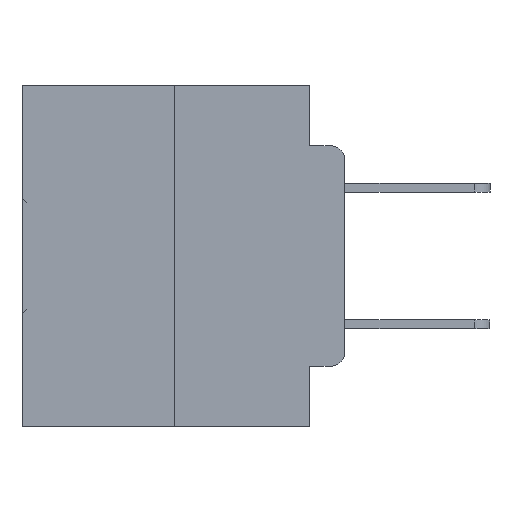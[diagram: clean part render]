
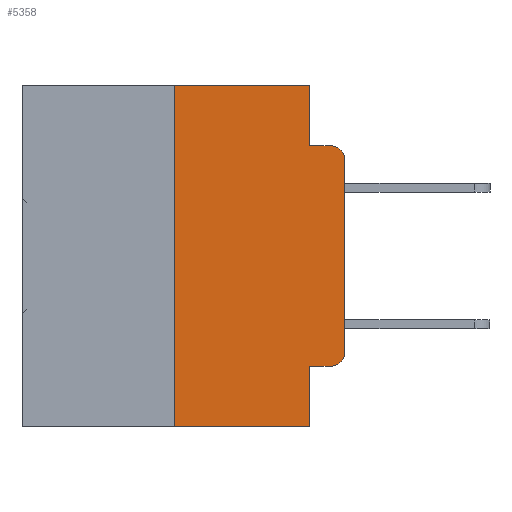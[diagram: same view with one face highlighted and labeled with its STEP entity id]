
A CAD part, left-side view. The second image highlights one B-rep face of the part: STEP entity #5358.
In plain terms, the highlighted planar face has unit normal (-1, 0, 0).
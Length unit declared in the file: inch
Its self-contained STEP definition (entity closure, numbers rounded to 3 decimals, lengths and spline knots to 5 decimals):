
#690 = CARTESIAN_POINT ( 'NONE',  ( 0., 0.051, -0.4115 ) ) ;
#1845 = DIRECTION ( 'NONE',  ( 0., -1., 0. ) ) ;
#2079 = CARTESIAN_POINT ( 'NONE',  ( 0., 0.25, -0.5 ) ) ;
#2485 = ORIENTED_EDGE ( 'NONE', *, *, #14139, .T. ) ;
#2536 = DIRECTION ( 'NONE',  ( 1., 0., 0. ) ) ;
#2561 = VERTEX_POINT ( 'NONE', #8249 ) ;
#4065 = LINE ( 'NONE', #8374, #10521 ) ;
#4293 = DIRECTION ( 'NONE',  ( 0., 0., 1. ) ) ;
#5358 = ADVANCED_FACE ( 'NONE', ( #15843 ), #18816, .F. ) ;
#5550 = AXIS2_PLACEMENT_3D ( 'NONE', #29505, #2536, #21541 ) ;
#5890 = CARTESIAN_POINT ( 'NONE',  ( 0., 0.051, -0.0885 ) ) ;
#6060 = EDGE_CURVE ( 'NONE', #31993, #30257, #15379, .T. ) ;
#6464 = VERTEX_POINT ( 'NONE', #7385 ) ;
#7130 = CIRCLE ( 'NONE', #8031, 0.02 ) ;
#7385 = CARTESIAN_POINT ( 'NONE',  ( 0., 0.051, -0.5 ) ) ;
#7533 = VECTOR ( 'NONE', #12114, 39.37008 ) ;
#8031 = AXIS2_PLACEMENT_3D ( 'NONE', #27682, #11628, #30417 ) ;
#8249 = CARTESIAN_POINT ( 'NONE',  ( 0., 0.02, -0.4115 ) ) ;
#8374 = CARTESIAN_POINT ( 'NONE',  ( 0., 0.473, 0. ) ) ;
#8397 = LINE ( 'NONE', #14814, #7533 ) ;
#8504 = ORIENTED_EDGE ( 'NONE', *, *, #6060, .F. ) ;
#9552 = EDGE_CURVE ( 'NONE', #32335, #24840, #14084, .T. ) ;
#10448 = EDGE_CURVE ( 'NONE', #24156, #6464, #14868, .T. ) ;
#10521 = VECTOR ( 'NONE', #29969, 39.37008 ) ;
#11304 = CARTESIAN_POINT ( 'NONE',  ( 0., 0.25, 0. ) ) ;
#11628 = DIRECTION ( 'NONE',  ( -1., 0., 0. ) ) ;
#11747 = CARTESIAN_POINT ( 'NONE',  ( 0., 0.02, -0.1085 ) ) ;
#11775 = AXIS2_PLACEMENT_3D ( 'NONE', #11747, #30529, #14446 ) ;
#11780 = VERTEX_POINT ( 'NONE', #16241 ) ;
#11903 = CARTESIAN_POINT ( 'NONE',  ( 0., 0.051, 0. ) ) ;
#12114 = DIRECTION ( 'NONE',  ( 0., 0., -1. ) ) ;
#12718 = CARTESIAN_POINT ( 'NONE',  ( 0., 0., 0. ) ) ;
#14007 = DIRECTION ( 'NONE',  ( 0., 0., 1. ) ) ;
#14016 = CARTESIAN_POINT ( 'NONE',  ( 0., 0., -0.1085 ) ) ;
#14084 = LINE ( 'NONE', #20851, #34625 ) ;
#14139 = EDGE_CURVE ( 'NONE', #20194, #27164, #27593, .T. ) ;
#14446 = DIRECTION ( 'NONE',  ( 0., 0., -1. ) ) ;
#14524 = ORIENTED_EDGE ( 'NONE', *, *, #17214, .T. ) ;
#14561 = VECTOR ( 'NONE', #33885, 39.37008 ) ;
#14765 = EDGE_CURVE ( 'NONE', #24156, #2561, #21674, .T. ) ;
#14814 = CARTESIAN_POINT ( 'NONE',  ( 0., 0.051, 0. ) ) ;
#14868 = LINE ( 'NONE', #11903, #29979 ) ;
#15379 = LINE ( 'NONE', #11304, #22541 ) ;
#15843 = FACE_OUTER_BOUND ( 'NONE', #30487, .T. ) ;
#16241 = CARTESIAN_POINT ( 'NONE',  ( 0., 0.051, 0. ) ) ;
#17214 = EDGE_CURVE ( 'NONE', #2561, #20194, #7130, .T. ) ;
#17261 = EDGE_CURVE ( 'NONE', #27164, #24840, #27839, .T. ) ;
#17443 = ORIENTED_EDGE ( 'NONE', *, *, #21713, .T. ) ;
#17823 = DIRECTION ( 'NONE',  ( 0., -1., 0. ) ) ;
#18374 = EDGE_CURVE ( 'NONE', #30257, #11780, #4065, .T. ) ;
#18658 = ORIENTED_EDGE ( 'NONE', *, *, #9552, .F. ) ;
#18816 = PLANE ( 'NONE',  #5550 ) ;
#20194 = VERTEX_POINT ( 'NONE', #26821 ) ;
#20476 = VECTOR ( 'NONE', #4293, 39.37008 ) ;
#20851 = CARTESIAN_POINT ( 'NONE',  ( 0., 0.051, -0.0885 ) ) ;
#21541 = DIRECTION ( 'NONE',  ( 0., 0., -1. ) ) ;
#21674 = LINE ( 'NONE', #31210, #14561 ) ;
#21713 = EDGE_CURVE ( 'NONE', #31993, #6464, #34153, .T. ) ;
#22064 = ORIENTED_EDGE ( 'NONE', *, *, #18374, .F. ) ;
#22541 = VECTOR ( 'NONE', #14007, 39.37008 ) ;
#22568 = DIRECTION ( 'NONE',  ( 0., 0., -1. ) ) ;
#24142 = ORIENTED_EDGE ( 'NONE', *, *, #17261, .T. ) ;
#24156 = VERTEX_POINT ( 'NONE', #690 ) ;
#24840 = VERTEX_POINT ( 'NONE', #33296 ) ;
#26632 = ORIENTED_EDGE ( 'NONE', *, *, #33195, .F. ) ;
#26821 = CARTESIAN_POINT ( 'NONE',  ( 0., 0., -0.3915 ) ) ;
#27164 = VERTEX_POINT ( 'NONE', #14016 ) ;
#27593 = LINE ( 'NONE', #12718, #20476 ) ;
#27682 = CARTESIAN_POINT ( 'NONE',  ( 0., 0.02, -0.3915 ) ) ;
#27839 = CIRCLE ( 'NONE', #11775, 0.02 ) ;
#27926 = ORIENTED_EDGE ( 'NONE', *, *, #14765, .T. ) ;
#29505 = CARTESIAN_POINT ( 'NONE',  ( 0., 0.473, 0. ) ) ;
#29969 = DIRECTION ( 'NONE',  ( 0., -1., 0. ) ) ;
#29979 = VECTOR ( 'NONE', #22568, 39.37008 ) ;
#30257 = VERTEX_POINT ( 'NONE', #30896 ) ;
#30417 = DIRECTION ( 'NONE',  ( 0., 0., -1. ) ) ;
#30487 = EDGE_LOOP ( 'NONE', ( #2485, #24142, #18658, #26632, #22064, #8504, #17443, #32542, #27926, #14524 ) ) ;
#30529 = DIRECTION ( 'NONE',  ( -1., 0., 0. ) ) ;
#30896 = CARTESIAN_POINT ( 'NONE',  ( 0., 0.25, 0. ) ) ;
#31210 = CARTESIAN_POINT ( 'NONE',  ( 0., 0.051, -0.4115 ) ) ;
#31236 = CARTESIAN_POINT ( 'NONE',  ( 0., 0.473, -0.5 ) ) ;
#31993 = VERTEX_POINT ( 'NONE', #2079 ) ;
#32335 = VERTEX_POINT ( 'NONE', #5890 ) ;
#32542 = ORIENTED_EDGE ( 'NONE', *, *, #10448, .F. ) ;
#33195 = EDGE_CURVE ( 'NONE', #11780, #32335, #8397, .T. ) ;
#33296 = CARTESIAN_POINT ( 'NONE',  ( 0., 0.02, -0.0885 ) ) ;
#33328 = VECTOR ( 'NONE', #17823, 39.37008 ) ;
#33885 = DIRECTION ( 'NONE',  ( 0., -1., 0. ) ) ;
#34153 = LINE ( 'NONE', #31236, #33328 ) ;
#34625 = VECTOR ( 'NONE', #1845, 39.37008 ) ;
